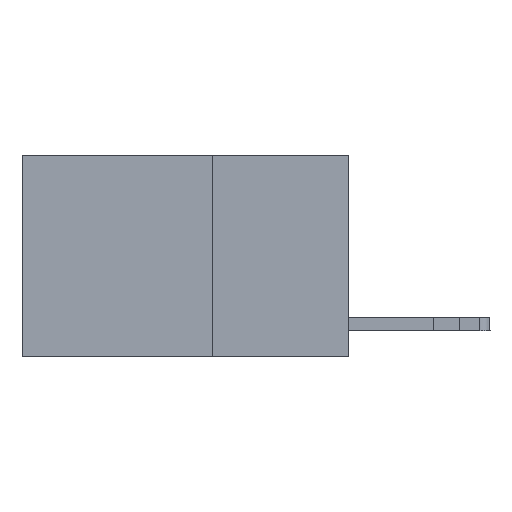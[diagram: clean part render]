
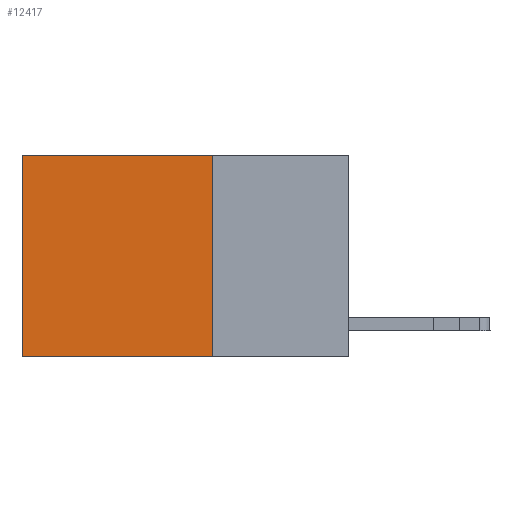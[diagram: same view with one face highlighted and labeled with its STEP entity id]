
A CAD part, left-side view. The second image highlights one B-rep face of the part: STEP entity #12417.
In plain terms, the highlighted planar face has unit normal (-1, 0, 0).
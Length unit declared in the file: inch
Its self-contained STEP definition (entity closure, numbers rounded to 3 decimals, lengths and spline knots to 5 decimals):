
#194 = VERTEX_POINT ( 'NONE', #8983 ) ;
#363 = EDGE_CURVE ( 'NONE', #10120, #1515, #11708, .T. ) ;
#586 = VECTOR ( 'NONE', #15568, 39.37008 ) ;
#1130 = CARTESIAN_POINT ( 'NONE',  ( 0.2625, 0.25, 0. ) ) ;
#1440 = VECTOR ( 'NONE', #7569, 39.37008 ) ;
#1515 = VERTEX_POINT ( 'NONE', #4550 ) ;
#1596 = CARTESIAN_POINT ( 'NONE',  ( 0.2625, 0.25, 0. ) ) ;
#4550 = CARTESIAN_POINT ( 'NONE',  ( 0.2625, 0.6, 0. ) ) ;
#5924 = CARTESIAN_POINT ( 'NONE',  ( 0.2625, 0.25, 0. ) ) ;
#6824 = PLANE ( 'NONE',  #8518 ) ;
#7309 = ORIENTED_EDGE ( 'NONE', *, *, #10560, .F. ) ;
#7354 = CARTESIAN_POINT ( 'NONE',  ( 0.2625, 0.25, 0. ) ) ;
#7569 = DIRECTION ( 'NONE',  ( 0., 0., -1. ) ) ;
#7866 = EDGE_CURVE ( 'NONE', #17449, #194, #9540, .T. ) ;
#8053 = DIRECTION ( 'NONE',  ( 0., 1., 0. ) ) ;
#8371 = CARTESIAN_POINT ( 'NONE',  ( 0.2625, 0.25, -0.37 ) ) ;
#8385 = CARTESIAN_POINT ( 'NONE',  ( 0.2625, 0.25, -0.37 ) ) ;
#8518 = AXIS2_PLACEMENT_3D ( 'NONE', #1596, #17000, #22128 ) ;
#8968 = VECTOR ( 'NONE', #12264, 39.37008 ) ;
#8983 = CARTESIAN_POINT ( 'NONE',  ( 0.2625, 0.6, -0.37 ) ) ;
#9540 = LINE ( 'NONE', #8371, #586 ) ;
#10120 = VERTEX_POINT ( 'NONE', #5924 ) ;
#10444 = EDGE_CURVE ( 'NONE', #1515, #194, #22332, .T. ) ;
#10560 = EDGE_CURVE ( 'NONE', #10120, #17449, #17648, .T. ) ;
#11708 = LINE ( 'NONE', #1130, #19391 ) ;
#11974 = ORIENTED_EDGE ( 'NONE', *, *, #7866, .F. ) ;
#12264 = DIRECTION ( 'NONE',  ( 0., 0., -1. ) ) ;
#12417 = ADVANCED_FACE ( 'NONE', ( #22472 ), #6824, .F. ) ;
#15568 = DIRECTION ( 'NONE',  ( 0., 1., 0. ) ) ;
#17000 = DIRECTION ( 'NONE',  ( 1., 0., 0. ) ) ;
#17314 = CARTESIAN_POINT ( 'NONE',  ( 0.2625, 0.6, 0. ) ) ;
#17449 = VERTEX_POINT ( 'NONE', #8385 ) ;
#17648 = LINE ( 'NONE', #7354, #1440 ) ;
#19183 = ORIENTED_EDGE ( 'NONE', *, *, #363, .T. ) ;
#19391 = VECTOR ( 'NONE', #8053, 39.37008 ) ;
#22128 = DIRECTION ( 'NONE',  ( 0., 0., -1. ) ) ;
#22158 = EDGE_LOOP ( 'NONE', ( #22426, #11974, #7309, #19183 ) ) ;
#22332 = LINE ( 'NONE', #17314, #8968 ) ;
#22426 = ORIENTED_EDGE ( 'NONE', *, *, #10444, .T. ) ;
#22472 = FACE_OUTER_BOUND ( 'NONE', #22158, .T. ) ;
